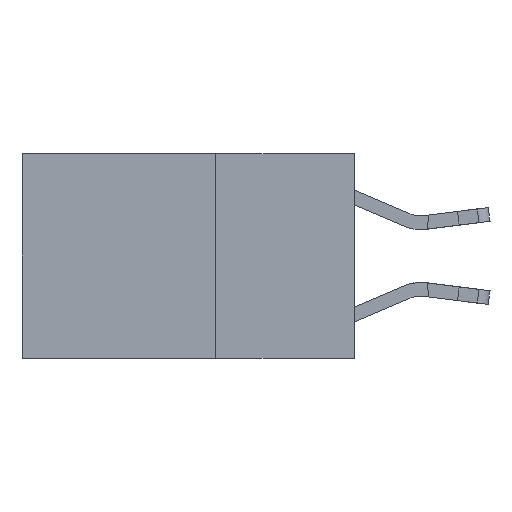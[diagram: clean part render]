
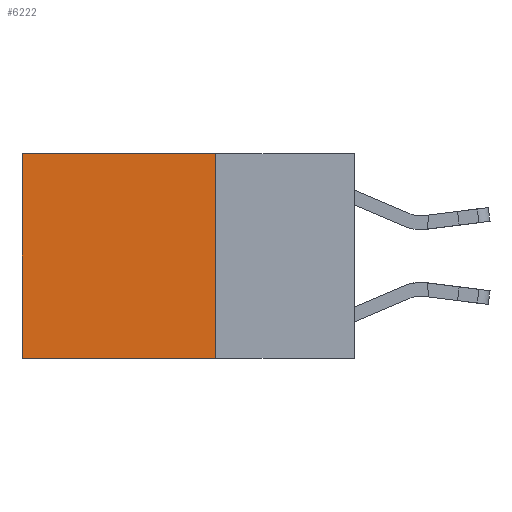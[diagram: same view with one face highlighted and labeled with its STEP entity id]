
A CAD part, left-side view. The second image highlights one B-rep face of the part: STEP entity #6222.
In plain terms, the highlighted planar face has unit normal (-1, 0, 0).
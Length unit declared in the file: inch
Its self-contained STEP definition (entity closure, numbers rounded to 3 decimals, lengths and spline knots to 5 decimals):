
#226 = FACE_OUTER_BOUND ( 'NONE', #10672, .T. ) ;
#2225 = DIRECTION ( 'NONE',  ( 0., 0., -1. ) ) ;
#3374 = ORIENTED_EDGE ( 'NONE', *, *, #21940, .T. ) ;
#5092 = CARTESIAN_POINT ( 'NONE',  ( 0.2625, 0.6, -0.37 ) ) ;
#5224 = CARTESIAN_POINT ( 'NONE',  ( 0.2625, 0.25, 0. ) ) ;
#5667 = EDGE_CURVE ( 'NONE', #10125, #25398, #12956, .T. ) ;
#5706 = AXIS2_PLACEMENT_3D ( 'NONE', #19202, #21762, #2225 ) ;
#6222 = ADVANCED_FACE ( 'NONE', ( #226 ), #24179, .F. ) ;
#6395 = DIRECTION ( 'NONE',  ( 0., 1., 0. ) ) ;
#6654 = LINE ( 'NONE', #17215, #13585 ) ;
#7026 = ORIENTED_EDGE ( 'NONE', *, *, #5667, .F. ) ;
#8354 = VERTEX_POINT ( 'NONE', #23405 ) ;
#9217 = DIRECTION ( 'NONE',  ( 0., 1., 0. ) ) ;
#9904 = ORIENTED_EDGE ( 'NONE', *, *, #22357, .F. ) ;
#10125 = VERTEX_POINT ( 'NONE', #10812 ) ;
#10672 = EDGE_LOOP ( 'NONE', ( #21387, #7026, #9904, #3374 ) ) ;
#10812 = CARTESIAN_POINT ( 'NONE',  ( 0.2625, 0.25, -0.37 ) ) ;
#12956 = LINE ( 'NONE', #13243, #20783 ) ;
#13243 = CARTESIAN_POINT ( 'NONE',  ( 0.2625, 0.25, -0.37 ) ) ;
#13585 = VECTOR ( 'NONE', #23615, 39.37008 ) ;
#13750 = CARTESIAN_POINT ( 'NONE',  ( 0.2625, 0.25, 0. ) ) ;
#14013 = VERTEX_POINT ( 'NONE', #13750 ) ;
#17215 = CARTESIAN_POINT ( 'NONE',  ( 0.2625, 0.6, 0. ) ) ;
#17225 = VECTOR ( 'NONE', #9217, 39.37008 ) ;
#17889 = DIRECTION ( 'NONE',  ( 0., 0., -1. ) ) ;
#18031 = CARTESIAN_POINT ( 'NONE',  ( 0.2625, 0.25, 0. ) ) ;
#19202 = CARTESIAN_POINT ( 'NONE',  ( 0.2625, 0.25, 0. ) ) ;
#19511 = VECTOR ( 'NONE', #17889, 39.37008 ) ;
#20783 = VECTOR ( 'NONE', #6395, 39.37008 ) ;
#21387 = ORIENTED_EDGE ( 'NONE', *, *, #21747, .T. ) ;
#21747 = EDGE_CURVE ( 'NONE', #8354, #25398, #6654, .T. ) ;
#21762 = DIRECTION ( 'NONE',  ( 1., 0., 0. ) ) ;
#21940 = EDGE_CURVE ( 'NONE', #14013, #8354, #26501, .T. ) ;
#22307 = LINE ( 'NONE', #18031, #19511 ) ;
#22357 = EDGE_CURVE ( 'NONE', #14013, #10125, #22307, .T. ) ;
#23405 = CARTESIAN_POINT ( 'NONE',  ( 0.2625, 0.6, 0. ) ) ;
#23615 = DIRECTION ( 'NONE',  ( 0., 0., -1. ) ) ;
#24179 = PLANE ( 'NONE',  #5706 ) ;
#25398 = VERTEX_POINT ( 'NONE', #5092 ) ;
#26501 = LINE ( 'NONE', #5224, #17225 ) ;
